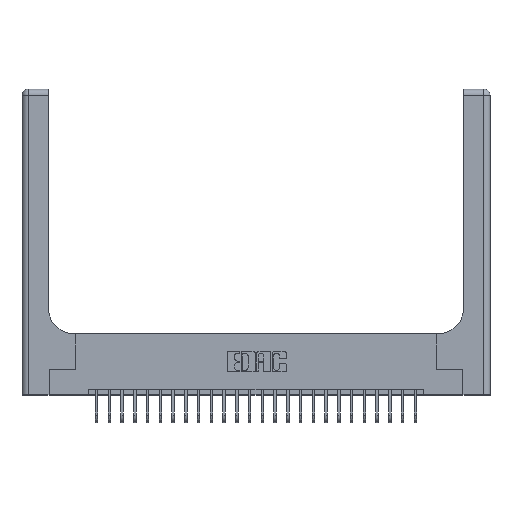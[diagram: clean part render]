
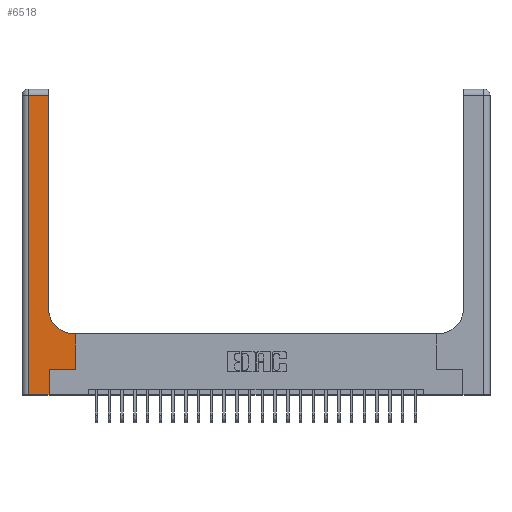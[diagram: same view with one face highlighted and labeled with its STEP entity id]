
A CAD part, top view. The second image highlights one B-rep face of the part: STEP entity #6518.
In plain terms, the highlighted planar face has unit normal (0, 0, 1).
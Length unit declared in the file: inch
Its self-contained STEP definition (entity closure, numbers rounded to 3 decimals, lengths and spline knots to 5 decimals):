
#115 = CARTESIAN_POINT ( 'NONE',  ( 0.528, 0.25, 0.37 ) ) ;
#153 = DIRECTION ( 'NONE',  ( 0., -1., 0. ) ) ;
#197 = CARTESIAN_POINT ( 'NONE',  ( 0.06, 0., 0.37 ) ) ;
#1231 = EDGE_CURVE ( 'NONE', #4073, #9058, #17943, .T. ) ;
#1359 = DIRECTION ( 'NONE',  ( 1., 0., 0. ) ) ;
#1940 = VERTEX_POINT ( 'NONE', #13360 ) ;
#2078 = CARTESIAN_POINT ( 'NONE',  ( 0.26, 0.85, 0.37 ) ) ;
#2341 = ORIENTED_EDGE ( 'NONE', *, *, #9629, .T. ) ;
#2532 = DIRECTION ( 'NONE',  ( 1., 0., 0. ) ) ;
#2537 = ORIENTED_EDGE ( 'NONE', *, *, #10264, .T. ) ;
#2651 = CARTESIAN_POINT ( 'NONE',  ( 0.26, 2.94, 0.37 ) ) ;
#2944 = ORIENTED_EDGE ( 'NONE', *, *, #11018, .T. ) ;
#3225 = ORIENTED_EDGE ( 'NONE', *, *, #10187, .T. ) ;
#3328 = LINE ( 'NONE', #19902, #22130 ) ;
#3371 = AXIS2_PLACEMENT_3D ( 'NONE', #20023, #9114, #21819 ) ;
#3577 = PLANE ( 'NONE',  #3371 ) ;
#3626 = VERTEX_POINT ( 'NONE', #115 ) ;
#3764 = ORIENTED_EDGE ( 'NONE', *, *, #1231, .T. ) ;
#4073 = VERTEX_POINT ( 'NONE', #18022 ) ;
#6057 = LINE ( 'NONE', #23143, #14622 ) ;
#6518 = ADVANCED_FACE ( 'NONE', ( #14894 ), #3577, .F. ) ;
#6810 = ORIENTED_EDGE ( 'NONE', *, *, #7980, .T. ) ;
#7090 = CARTESIAN_POINT ( 'NONE',  ( 0.51, 0.6, 0.37 ) ) ;
#7120 = VECTOR ( 'NONE', #153, 39.37008 ) ;
#7132 = VERTEX_POINT ( 'NONE', #7090 ) ;
#7980 = EDGE_CURVE ( 'NONE', #13113, #1940, #8231, .T. ) ;
#8231 = LINE ( 'NONE', #15024, #22167 ) ;
#8610 = EDGE_CURVE ( 'NONE', #9058, #13113, #14980, .T. ) ;
#9058 = VERTEX_POINT ( 'NONE', #197 ) ;
#9114 = DIRECTION ( 'NONE',  ( 0., 0., -1. ) ) ;
#9267 = CARTESIAN_POINT ( 'NONE',  ( 0.06, 3., 0.37 ) ) ;
#9283 = DIRECTION ( 'NONE',  ( 0., 0., -1. ) ) ;
#9462 = EDGE_LOOP ( 'NONE', ( #3225, #2944, #3764, #22200, #6810, #2537, #15467, #12349, #2341 ) ) ;
#9629 = EDGE_CURVE ( 'NONE', #7132, #18757, #23409, .T. ) ;
#10187 = EDGE_CURVE ( 'NONE', #18757, #18362, #20570, .T. ) ;
#10264 = EDGE_CURVE ( 'NONE', #1940, #3626, #6057, .T. ) ;
#10890 = LINE ( 'NONE', #15249, #19421 ) ;
#10894 = VECTOR ( 'NONE', #14367, 39.37008 ) ;
#11018 = EDGE_CURVE ( 'NONE', #18362, #4073, #14629, .T. ) ;
#12349 = ORIENTED_EDGE ( 'NONE', *, *, #14782, .T. ) ;
#13113 = VERTEX_POINT ( 'NONE', #22082 ) ;
#13360 = CARTESIAN_POINT ( 'NONE',  ( 0.265, 0.25, 0.37 ) ) ;
#14367 = DIRECTION ( 'NONE',  ( 0., 1., 0. ) ) ;
#14622 = VECTOR ( 'NONE', #1359, 39.37008 ) ;
#14629 = LINE ( 'NONE', #18533, #18862 ) ;
#14782 = EDGE_CURVE ( 'NONE', #14957, #7132, #3328, .T. ) ;
#14894 = FACE_OUTER_BOUND ( 'NONE', #9462, .T. ) ;
#14957 = VERTEX_POINT ( 'NONE', #18523 ) ;
#14980 = LINE ( 'NONE', #15310, #18645 ) ;
#15024 = CARTESIAN_POINT ( 'NONE',  ( 0.265, 0., 0.37 ) ) ;
#15249 = CARTESIAN_POINT ( 'NONE',  ( 0.528, 0.25, 0.37 ) ) ;
#15310 = CARTESIAN_POINT ( 'NONE',  ( 0., 0., 0.37 ) ) ;
#15467 = ORIENTED_EDGE ( 'NONE', *, *, #21932, .T. ) ;
#17059 = DIRECTION ( 'NONE',  ( 0., 1., 0. ) ) ;
#17943 = LINE ( 'NONE', #9267, #7120 ) ;
#18022 = CARTESIAN_POINT ( 'NONE',  ( 0.06, 2.94, 0.37 ) ) ;
#18362 = VERTEX_POINT ( 'NONE', #2651 ) ;
#18523 = CARTESIAN_POINT ( 'NONE',  ( 0.528, 0.6, 0.37 ) ) ;
#18533 = CARTESIAN_POINT ( 'NONE',  ( 0., 2.94, 0.37 ) ) ;
#18645 = VECTOR ( 'NONE', #2532, 39.37008 ) ;
#18646 = DIRECTION ( 'NONE',  ( 0., 1., 0. ) ) ;
#18757 = VERTEX_POINT ( 'NONE', #2078 ) ;
#18862 = VECTOR ( 'NONE', #20375, 39.37008 ) ;
#19421 = VECTOR ( 'NONE', #17059, 39.37008 ) ;
#19837 = CARTESIAN_POINT ( 'NONE',  ( 0.26, 3., 0.37 ) ) ;
#19902 = CARTESIAN_POINT ( 'NONE',  ( 0.26, 0.6, 0.37 ) ) ;
#20023 = CARTESIAN_POINT ( 'NONE',  ( 0., 3., 0.37 ) ) ;
#20181 = CARTESIAN_POINT ( 'NONE',  ( 0.51, 0.85, 0.37 ) ) ;
#20375 = DIRECTION ( 'NONE',  ( -1., 0., 0. ) ) ;
#20570 = LINE ( 'NONE', #19837, #10894 ) ;
#21705 = DIRECTION ( 'NONE',  ( -1., 0., 0. ) ) ;
#21819 = DIRECTION ( 'NONE',  ( -1., 0., 0. ) ) ;
#21932 = EDGE_CURVE ( 'NONE', #3626, #14957, #10890, .T. ) ;
#21981 = DIRECTION ( 'NONE',  ( 1., 0., 0. ) ) ;
#22082 = CARTESIAN_POINT ( 'NONE',  ( 0.265, 0., 0.37 ) ) ;
#22130 = VECTOR ( 'NONE', #21705, 39.37008 ) ;
#22167 = VECTOR ( 'NONE', #18646, 39.37008 ) ;
#22200 = ORIENTED_EDGE ( 'NONE', *, *, #8610, .T. ) ;
#22907 = AXIS2_PLACEMENT_3D ( 'NONE', #20181, #9283, #21981 ) ;
#23143 = CARTESIAN_POINT ( 'NONE',  ( 0.265, 0.25, 0.37 ) ) ;
#23409 = CIRCLE ( 'NONE', #22907, 0.25 ) ;
